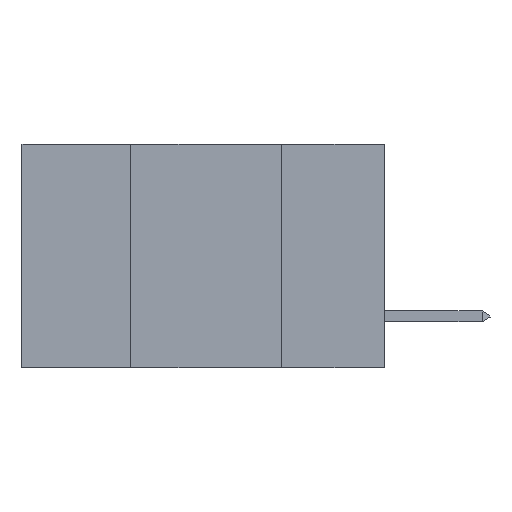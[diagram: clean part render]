
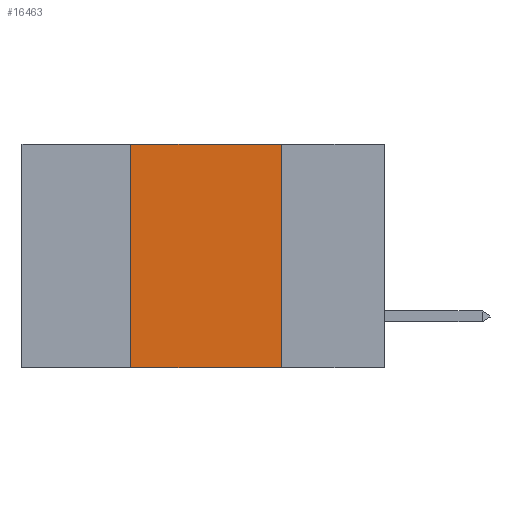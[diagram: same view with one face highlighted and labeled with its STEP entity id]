
A CAD part, left-side view. The second image highlights one B-rep face of the part: STEP entity #16463.
In plain terms, the highlighted planar face has unit normal (-1, 0, 0).
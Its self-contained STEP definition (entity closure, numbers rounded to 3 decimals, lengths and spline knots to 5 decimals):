
#1736 = CARTESIAN_POINT ( 'NONE',  ( 0., 0.17, -0.37 ) ) ;
#1789 = VECTOR ( 'NONE', #12325, 39.37008 ) ;
#4556 = DIRECTION ( 'NONE',  ( 0., 0., -1. ) ) ;
#5321 = LINE ( 'NONE', #13306, #16502 ) ;
#5932 = VECTOR ( 'NONE', #45849, 39.37008 ) ;
#8720 = CARTESIAN_POINT ( 'NONE',  ( 0., 0.42, 0. ) ) ;
#8814 = VERTEX_POINT ( 'NONE', #20195 ) ;
#8882 = AXIS2_PLACEMENT_3D ( 'NONE', #26828, #23246, #4556 ) ;
#12325 = DIRECTION ( 'NONE',  ( 0., -1., 0. ) ) ;
#13011 = LINE ( 'NONE', #22593, #41159 ) ;
#13306 = CARTESIAN_POINT ( 'NONE',  ( 0., 0.42, 0. ) ) ;
#14255 = ORIENTED_EDGE ( 'NONE', *, *, #27350, .T. ) ;
#15696 = VERTEX_POINT ( 'NONE', #36204 ) ;
#16463 = ADVANCED_FACE ( 'NONE', ( #28938 ), #30590, .F. ) ;
#16502 = VECTOR ( 'NONE', #37183, 39.37008 ) ;
#20195 = CARTESIAN_POINT ( 'NONE',  ( 0., 0.42, -0.37 ) ) ;
#22593 = CARTESIAN_POINT ( 'NONE',  ( 0., 0.17, 0. ) ) ;
#23246 = DIRECTION ( 'NONE',  ( 1., 0., 0. ) ) ;
#25798 = LINE ( 'NONE', #42318, #1789 ) ;
#26006 = DIRECTION ( 'NONE',  ( 0., 0., -1. ) ) ;
#26828 = CARTESIAN_POINT ( 'NONE',  ( 0., 0.6, 0. ) ) ;
#27350 = EDGE_CURVE ( 'NONE', #8814, #42799, #28800, .T. ) ;
#28800 = LINE ( 'NONE', #41924, #5932 ) ;
#28938 = FACE_OUTER_BOUND ( 'NONE', #30029, .T. ) ;
#30029 = EDGE_LOOP ( 'NONE', ( #45924, #32116, #39863, #14255 ) ) ;
#30590 = PLANE ( 'NONE',  #8882 ) ;
#32116 = ORIENTED_EDGE ( 'NONE', *, *, #40278, .F. ) ;
#33151 = EDGE_CURVE ( 'NONE', #15696, #42799, #13011, .T. ) ;
#36204 = CARTESIAN_POINT ( 'NONE',  ( 0., 0.17, 0. ) ) ;
#37183 = DIRECTION ( 'NONE',  ( 0., 0., 1. ) ) ;
#39863 = ORIENTED_EDGE ( 'NONE', *, *, #45450, .F. ) ;
#40203 = VERTEX_POINT ( 'NONE', #8720 ) ;
#40278 = EDGE_CURVE ( 'NONE', #40203, #15696, #25798, .T. ) ;
#41159 = VECTOR ( 'NONE', #26006, 39.37008 ) ;
#41924 = CARTESIAN_POINT ( 'NONE',  ( 0., 0.6, -0.37 ) ) ;
#42318 = CARTESIAN_POINT ( 'NONE',  ( 0., 0.6, 0. ) ) ;
#42799 = VERTEX_POINT ( 'NONE', #1736 ) ;
#45450 = EDGE_CURVE ( 'NONE', #8814, #40203, #5321, .T. ) ;
#45849 = DIRECTION ( 'NONE',  ( 0., -1., 0. ) ) ;
#45924 = ORIENTED_EDGE ( 'NONE', *, *, #33151, .F. ) ;
